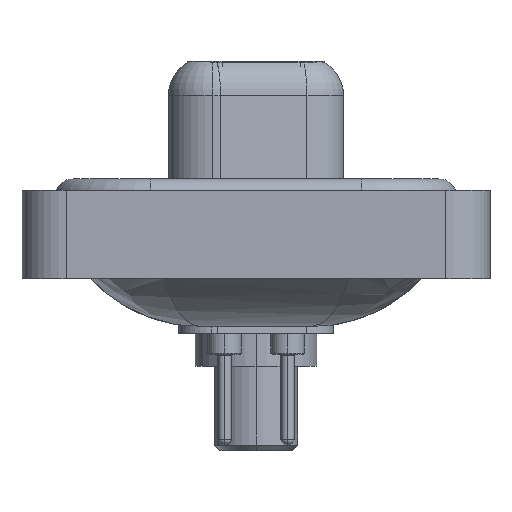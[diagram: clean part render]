
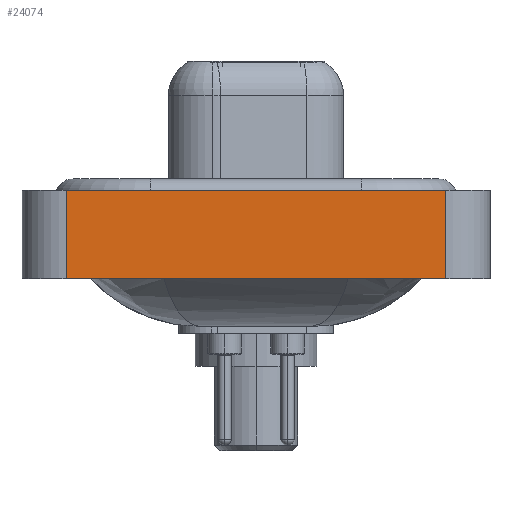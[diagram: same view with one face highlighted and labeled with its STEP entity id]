
A CAD part, left-side view. The second image highlights one B-rep face of the part: STEP entity #24074.
In plain terms, the highlighted planar face has unit normal (-1, 0, 0).
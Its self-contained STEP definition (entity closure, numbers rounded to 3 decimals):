
#392 = ORIENTED_EDGE ( 'NONE', *, *, #23079, .T. ) ;
#727 = EDGE_CURVE ( 'NONE', #18897, #7876, #3554, .T. ) ;
#963 = ORIENTED_EDGE ( 'NONE', *, *, #1802, .T. ) ;
#1340 = DIRECTION ( 'NONE',  ( 0., 0., 1. ) ) ;
#1582 = DIRECTION ( 'NONE',  ( 0., 0., 1. ) ) ;
#1802 = EDGE_CURVE ( 'NONE', #8766, #8287, #12593, .T. ) ;
#3377 = DIRECTION ( 'NONE',  ( 0., -1., 0. ) ) ;
#3554 = LINE ( 'NONE', #19688, #5315 ) ;
#5315 = VECTOR ( 'NONE', #1582, 1000. ) ;
#5427 = FACE_OUTER_BOUND ( 'NONE', #8994, .T. ) ;
#5811 = ORIENTED_EDGE ( 'NONE', *, *, #727, .F. ) ;
#7142 = LINE ( 'NONE', #23230, #23633 ) ;
#7697 = CARTESIAN_POINT ( 'NONE',  ( -7.35, -8.55, -3.6 ) ) ;
#7876 = VERTEX_POINT ( 'NONE', #12044 ) ;
#8287 = VERTEX_POINT ( 'NONE', #14605 ) ;
#8617 = DIRECTION ( 'NONE',  ( 0., 0., 1. ) ) ;
#8759 = VECTOR ( 'NONE', #8617, 1000. ) ;
#8766 = VERTEX_POINT ( 'NONE', #16902 ) ;
#8994 = EDGE_LOOP ( 'NONE', ( #963, #23747, #5811, #392 ) ) ;
#9199 = CARTESIAN_POINT ( 'NONE',  ( -7.35, 8.55, -3.6 ) ) ;
#11401 = DIRECTION ( 'NONE',  ( -1., 0., 0. ) ) ;
#12016 = EDGE_CURVE ( 'NONE', #7876, #8287, #13311, .T. ) ;
#12044 = CARTESIAN_POINT ( 'NONE',  ( -7.35, 8.55, 0.4 ) ) ;
#12593 = LINE ( 'NONE', #18652, #8759 ) ;
#13311 = LINE ( 'NONE', #21353, #18242 ) ;
#14605 = CARTESIAN_POINT ( 'NONE',  ( -7.35, -8.55, 0.4 ) ) ;
#16902 = CARTESIAN_POINT ( 'NONE',  ( -7.35, -8.55, -3.6 ) ) ;
#18242 = VECTOR ( 'NONE', #3377, 1000. ) ;
#18652 = CARTESIAN_POINT ( 'NONE',  ( -7.35, -8.55, -3.6 ) ) ;
#18897 = VERTEX_POINT ( 'NONE', #9199 ) ;
#19580 = PLANE ( 'NONE',  #23287 ) ;
#19688 = CARTESIAN_POINT ( 'NONE',  ( -7.35, 8.55, -3.6 ) ) ;
#21271 = DIRECTION ( 'NONE',  ( 0., -1., 0. ) ) ;
#21353 = CARTESIAN_POINT ( 'NONE',  ( -7.35, -8.55, 0.4 ) ) ;
#23079 = EDGE_CURVE ( 'NONE', #18897, #8766, #7142, .T. ) ;
#23230 = CARTESIAN_POINT ( 'NONE',  ( -7.35, -8.55, -3.6 ) ) ;
#23287 = AXIS2_PLACEMENT_3D ( 'NONE', #7697, #11401, #1340 ) ;
#23633 = VECTOR ( 'NONE', #21271, 1000. ) ;
#23747 = ORIENTED_EDGE ( 'NONE', *, *, #12016, .F. ) ;
#24074 = ADVANCED_FACE ( 'NONE', ( #5427 ), #19580, .T. ) ;
